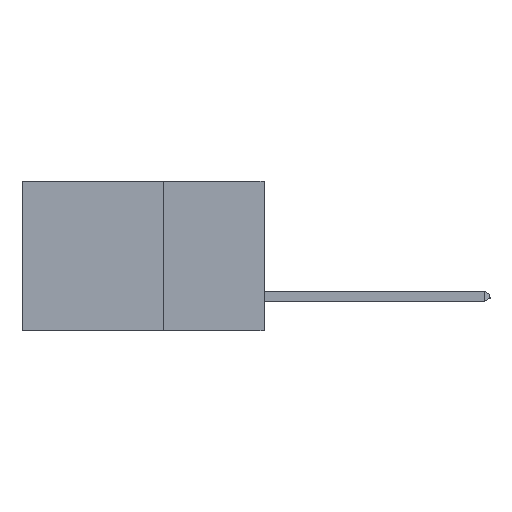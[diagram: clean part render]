
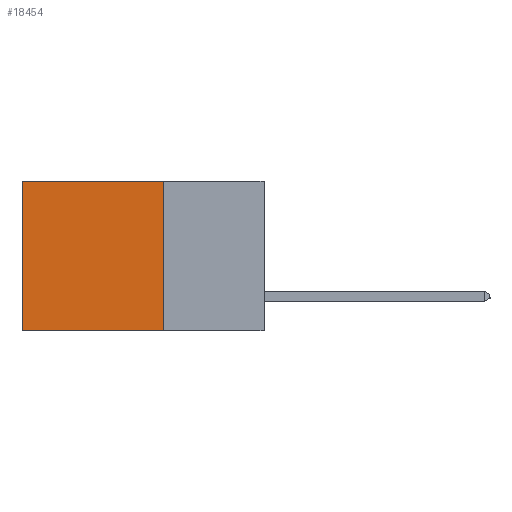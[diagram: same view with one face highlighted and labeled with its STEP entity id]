
A CAD part, left-side view. The second image highlights one B-rep face of the part: STEP entity #18454.
In plain terms, the highlighted planar face has unit normal (-1, 0, 0).
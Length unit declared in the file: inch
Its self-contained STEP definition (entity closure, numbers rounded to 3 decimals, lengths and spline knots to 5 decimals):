
#694 = DIRECTION ( 'NONE',  ( 0., 0., -1. ) ) ;
#775 = VERTEX_POINT ( 'NONE', #15552 ) ;
#786 = DIRECTION ( 'NONE',  ( 0., 0., -1. ) ) ;
#1071 = CARTESIAN_POINT ( 'NONE',  ( 0.298, 0.25, 0. ) ) ;
#3556 = FACE_OUTER_BOUND ( 'NONE', #5820, .T. ) ;
#3673 = LINE ( 'NONE', #10430, #14368 ) ;
#4324 = LINE ( 'NONE', #9337, #11987 ) ;
#4383 = VECTOR ( 'NONE', #694, 39.37008 ) ;
#4524 = VERTEX_POINT ( 'NONE', #7555 ) ;
#4704 = EDGE_CURVE ( 'NONE', #15726, #775, #12506, .T. ) ;
#5729 = VECTOR ( 'NONE', #12821, 39.37008 ) ;
#5820 = EDGE_LOOP ( 'NONE', ( #16466, #15502, #15167, #13416 ) ) ;
#6104 = EDGE_CURVE ( 'NONE', #15726, #4524, #4324, .T. ) ;
#6206 = LINE ( 'NONE', #11317, #5729 ) ;
#7555 = CARTESIAN_POINT ( 'NONE',  ( 0.298, 0.6, 0. ) ) ;
#7923 = CARTESIAN_POINT ( 'NONE',  ( 0.298, 0.25, 0. ) ) ;
#8476 = PLANE ( 'NONE',  #14701 ) ;
#9337 = CARTESIAN_POINT ( 'NONE',  ( 0.298, 0.25, 0. ) ) ;
#9514 = DIRECTION ( 'NONE',  ( 0., 1., 0. ) ) ;
#10013 = DIRECTION ( 'NONE',  ( 1., 0., 0. ) ) ;
#10430 = CARTESIAN_POINT ( 'NONE',  ( 0.298, 0.25, -0.37 ) ) ;
#11317 = CARTESIAN_POINT ( 'NONE',  ( 0.298, 0.6, 0. ) ) ;
#11987 = VECTOR ( 'NONE', #9514, 39.37008 ) ;
#12506 = LINE ( 'NONE', #1071, #4383 ) ;
#12604 = CARTESIAN_POINT ( 'NONE',  ( 0.298, 0.6, -0.37 ) ) ;
#12821 = DIRECTION ( 'NONE',  ( 0., 0., -1. ) ) ;
#13416 = ORIENTED_EDGE ( 'NONE', *, *, #6104, .T. ) ;
#13497 = DIRECTION ( 'NONE',  ( 0., 1., 0. ) ) ;
#14368 = VECTOR ( 'NONE', #13497, 39.37008 ) ;
#14701 = AXIS2_PLACEMENT_3D ( 'NONE', #18807, #10013, #786 ) ;
#15167 = ORIENTED_EDGE ( 'NONE', *, *, #4704, .F. ) ;
#15427 = EDGE_CURVE ( 'NONE', #775, #15761, #3673, .T. ) ;
#15502 = ORIENTED_EDGE ( 'NONE', *, *, #15427, .F. ) ;
#15552 = CARTESIAN_POINT ( 'NONE',  ( 0.298, 0.25, -0.37 ) ) ;
#15726 = VERTEX_POINT ( 'NONE', #7923 ) ;
#15761 = VERTEX_POINT ( 'NONE', #12604 ) ;
#16466 = ORIENTED_EDGE ( 'NONE', *, *, #18355, .T. ) ;
#18355 = EDGE_CURVE ( 'NONE', #4524, #15761, #6206, .T. ) ;
#18454 = ADVANCED_FACE ( 'NONE', ( #3556 ), #8476, .F. ) ;
#18807 = CARTESIAN_POINT ( 'NONE',  ( 0.298, 0.25, 0. ) ) ;
